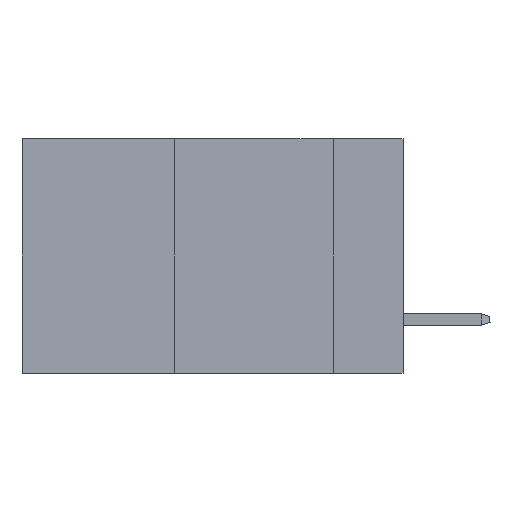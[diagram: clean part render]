
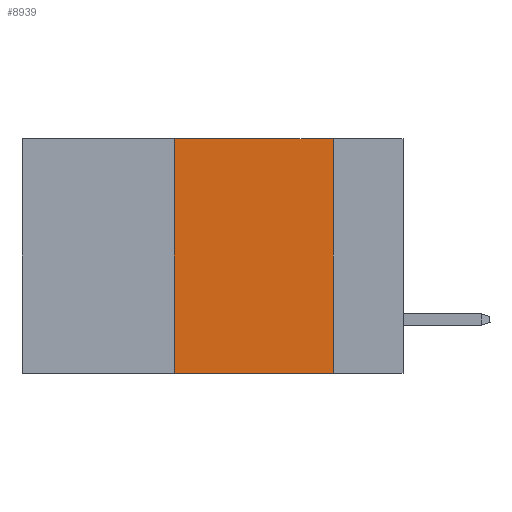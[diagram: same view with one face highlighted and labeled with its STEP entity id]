
A CAD part, left-side view. The second image highlights one B-rep face of the part: STEP entity #8939.
In plain terms, the highlighted planar face has unit normal (-1, 0, 0).
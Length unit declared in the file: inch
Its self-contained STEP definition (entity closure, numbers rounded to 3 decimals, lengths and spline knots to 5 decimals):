
#1282 = ORIENTED_EDGE ( 'NONE', *, *, #4162, .T. ) ;
#2401 = ORIENTED_EDGE ( 'NONE', *, *, #19612, .F. ) ;
#3371 = FACE_OUTER_BOUND ( 'NONE', #3797, .T. ) ;
#3455 = CARTESIAN_POINT ( 'NONE',  ( 0., 0.11, 0. ) ) ;
#3797 = EDGE_LOOP ( 'NONE', ( #3928, #23217, #2401, #1282 ) ) ;
#3928 = ORIENTED_EDGE ( 'NONE', *, *, #22376, .F. ) ;
#4064 = LINE ( 'NONE', #15608, #11027 ) ;
#4162 = EDGE_CURVE ( 'NONE', #10509, #19707, #10176, .T. ) ;
#4486 = EDGE_CURVE ( 'NONE', #22016, #10832, #4064, .T. ) ;
#5605 = PLANE ( 'NONE',  #16222 ) ;
#5714 = CARTESIAN_POINT ( 'NONE',  ( 0., 0.11, 0. ) ) ;
#8387 = CARTESIAN_POINT ( 'NONE',  ( 0., 0.36, -0.37 ) ) ;
#8432 = VECTOR ( 'NONE', #21022, 39.37008 ) ;
#8939 = ADVANCED_FACE ( 'NONE', ( #3371 ), #5605, .F. ) ;
#9217 = CARTESIAN_POINT ( 'NONE',  ( 0., 0.6, 0. ) ) ;
#9430 = LINE ( 'NONE', #3455, #21275 ) ;
#10176 = LINE ( 'NONE', #22001, #18769 ) ;
#10405 = CARTESIAN_POINT ( 'NONE',  ( 0., 0.36, 0. ) ) ;
#10509 = VERTEX_POINT ( 'NONE', #8387 ) ;
#10832 = VERTEX_POINT ( 'NONE', #5714 ) ;
#11027 = VECTOR ( 'NONE', #22112, 39.37008 ) ;
#11926 = DIRECTION ( 'NONE',  ( 0., -1., 0. ) ) ;
#12409 = LINE ( 'NONE', #10405, #8432 ) ;
#13728 = DIRECTION ( 'NONE',  ( 1., 0., 0. ) ) ;
#15608 = CARTESIAN_POINT ( 'NONE',  ( 0., 0.6, 0. ) ) ;
#16222 = AXIS2_PLACEMENT_3D ( 'NONE', #9217, #13728, #19806 ) ;
#18742 = CARTESIAN_POINT ( 'NONE',  ( 0., 0.11, -0.37 ) ) ;
#18769 = VECTOR ( 'NONE', #11926, 39.37008 ) ;
#19612 = EDGE_CURVE ( 'NONE', #10509, #22016, #12409, .T. ) ;
#19707 = VERTEX_POINT ( 'NONE', #18742 ) ;
#19806 = DIRECTION ( 'NONE',  ( 0., 0., -1. ) ) ;
#20282 = DIRECTION ( 'NONE',  ( 0., 0., -1. ) ) ;
#20588 = CARTESIAN_POINT ( 'NONE',  ( 0., 0.36, 0. ) ) ;
#21022 = DIRECTION ( 'NONE',  ( 0., 0., 1. ) ) ;
#21275 = VECTOR ( 'NONE', #20282, 39.37008 ) ;
#22001 = CARTESIAN_POINT ( 'NONE',  ( 0., 0.6, -0.37 ) ) ;
#22016 = VERTEX_POINT ( 'NONE', #20588 ) ;
#22112 = DIRECTION ( 'NONE',  ( 0., -1., 0. ) ) ;
#22376 = EDGE_CURVE ( 'NONE', #10832, #19707, #9430, .T. ) ;
#23217 = ORIENTED_EDGE ( 'NONE', *, *, #4486, .F. ) ;
